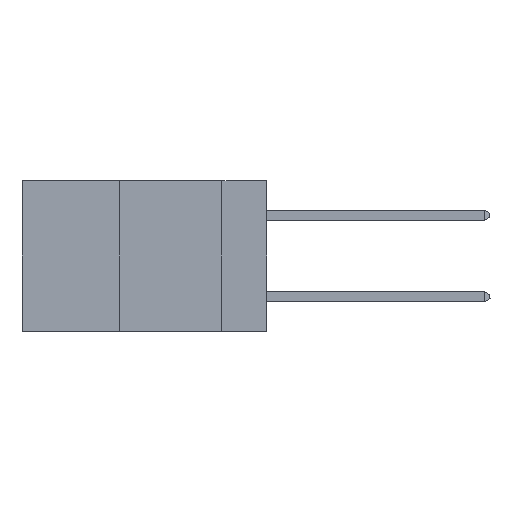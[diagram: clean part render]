
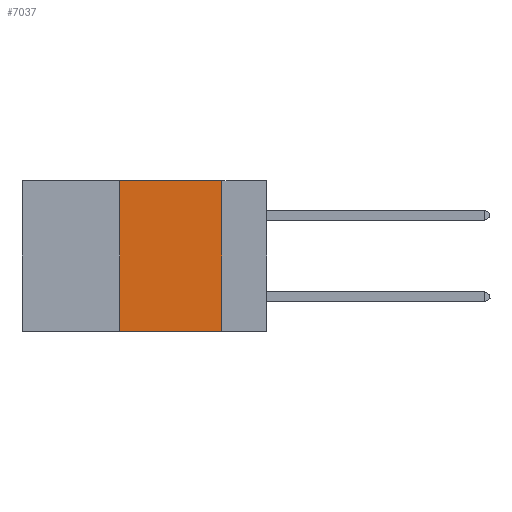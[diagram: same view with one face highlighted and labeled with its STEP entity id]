
A CAD part, left-side view. The second image highlights one B-rep face of the part: STEP entity #7037.
In plain terms, the highlighted planar face has unit normal (-1, 0, 0).
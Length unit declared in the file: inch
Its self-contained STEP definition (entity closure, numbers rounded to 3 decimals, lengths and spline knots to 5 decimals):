
#756 = VERTEX_POINT ( 'NONE', #9362 ) ;
#1186 = LINE ( 'NONE', #5471, #2768 ) ;
#2438 = LINE ( 'NONE', #17317, #10562 ) ;
#2502 = EDGE_CURVE ( 'NONE', #18462, #15013, #18118, .T. ) ;
#2768 = VECTOR ( 'NONE', #19547, 39.37008 ) ;
#3365 = DIRECTION ( 'NONE',  ( 0., 0., 1. ) ) ;
#4358 = CARTESIAN_POINT ( 'NONE',  ( 0., 0.11, 0. ) ) ;
#5258 = CARTESIAN_POINT ( 'NONE',  ( 0., 0.6, 0. ) ) ;
#5471 = CARTESIAN_POINT ( 'NONE',  ( 0., 0.6, 0. ) ) ;
#5503 = VECTOR ( 'NONE', #11016, 39.37008 ) ;
#7037 = ADVANCED_FACE ( 'NONE', ( #13490 ), #13216, .F. ) ;
#7876 = ORIENTED_EDGE ( 'NONE', *, *, #2502, .F. ) ;
#8713 = EDGE_CURVE ( 'NONE', #20780, #756, #2438, .T. ) ;
#9343 = DIRECTION ( 'NONE',  ( 0., 0., -1. ) ) ;
#9362 = CARTESIAN_POINT ( 'NONE',  ( 0., 0.36, 0. ) ) ;
#9550 = CARTESIAN_POINT ( 'NONE',  ( 0., 0.6, -0.37 ) ) ;
#9837 = EDGE_LOOP ( 'NONE', ( #7876, #23216, #24638, #13048 ) ) ;
#10562 = VECTOR ( 'NONE', #3365, 39.37008 ) ;
#11016 = DIRECTION ( 'NONE',  ( 0., 0., -1. ) ) ;
#11959 = VECTOR ( 'NONE', #15729, 39.37008 ) ;
#13048 = ORIENTED_EDGE ( 'NONE', *, *, #18920, .T. ) ;
#13216 = PLANE ( 'NONE',  #25543 ) ;
#13490 = FACE_OUTER_BOUND ( 'NONE', #9837, .T. ) ;
#14075 = CARTESIAN_POINT ( 'NONE',  ( 0., 0.11, -0.37 ) ) ;
#15013 = VERTEX_POINT ( 'NONE', #14075 ) ;
#15729 = DIRECTION ( 'NONE',  ( 0., -1., 0. ) ) ;
#17317 = CARTESIAN_POINT ( 'NONE',  ( 0., 0.36, 0. ) ) ;
#18118 = LINE ( 'NONE', #22958, #5503 ) ;
#18462 = VERTEX_POINT ( 'NONE', #4358 ) ;
#18920 = EDGE_CURVE ( 'NONE', #20780, #15013, #19870, .T. ) ;
#19547 = DIRECTION ( 'NONE',  ( 0., -1., 0. ) ) ;
#19870 = LINE ( 'NONE', #9550, #11959 ) ;
#20266 = EDGE_CURVE ( 'NONE', #756, #18462, #1186, .T. ) ;
#20780 = VERTEX_POINT ( 'NONE', #23238 ) ;
#21130 = DIRECTION ( 'NONE',  ( 1., 0., 0. ) ) ;
#22958 = CARTESIAN_POINT ( 'NONE',  ( 0., 0.11, 0. ) ) ;
#23216 = ORIENTED_EDGE ( 'NONE', *, *, #20266, .F. ) ;
#23238 = CARTESIAN_POINT ( 'NONE',  ( 0., 0.36, -0.37 ) ) ;
#24638 = ORIENTED_EDGE ( 'NONE', *, *, #8713, .F. ) ;
#25543 = AXIS2_PLACEMENT_3D ( 'NONE', #5258, #21130, #9343 ) ;
